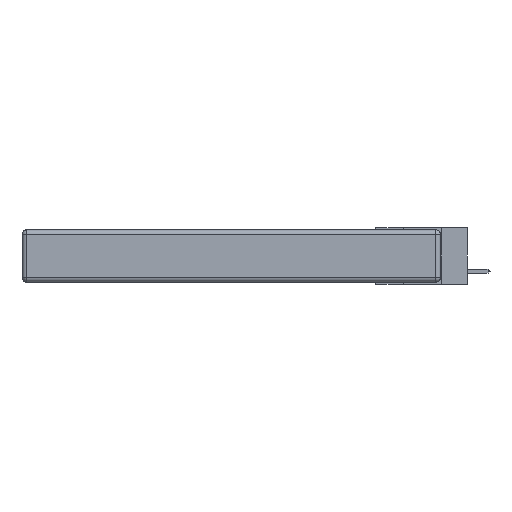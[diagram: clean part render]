
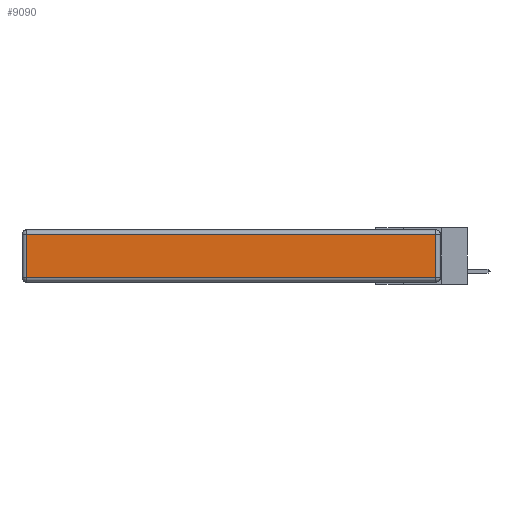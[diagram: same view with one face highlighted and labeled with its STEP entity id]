
A CAD part, left-side view. The second image highlights one B-rep face of the part: STEP entity #9090.
In plain terms, the highlighted planar face has unit normal (-1, 0, 0).
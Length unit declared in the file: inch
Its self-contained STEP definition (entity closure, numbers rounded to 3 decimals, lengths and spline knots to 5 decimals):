
#106 = CARTESIAN_POINT ( 'NONE',  ( 0., 0.03, -0.313 ) ) ;
#1104 = PLANE ( 'NONE',  #8546 ) ;
#1683 = CARTESIAN_POINT ( 'NONE',  ( 0., 2.75, -0.03 ) ) ;
#2024 = VECTOR ( 'NONE', #6876, 39.37008 ) ;
#2423 = FACE_OUTER_BOUND ( 'NONE', #12102, .T. ) ;
#2875 = CARTESIAN_POINT ( 'NONE',  ( 0., 0., -0.343 ) ) ;
#2910 = ORIENTED_EDGE ( 'NONE', *, *, #21826, .T. ) ;
#3122 = VECTOR ( 'NONE', #6326, 39.37008 ) ;
#3180 = LINE ( 'NONE', #3211, #18531 ) ;
#3211 = CARTESIAN_POINT ( 'NONE',  ( 0., 2.72, -0.343 ) ) ;
#3883 = CARTESIAN_POINT ( 'NONE',  ( 0., 2.72, -0.313 ) ) ;
#5077 = EDGE_CURVE ( 'NONE', #22896, #17038, #14555, .T. ) ;
#5767 = ORIENTED_EDGE ( 'NONE', *, *, #5077, .T. ) ;
#6326 = DIRECTION ( 'NONE',  ( 0., 0., 1. ) ) ;
#6363 = DIRECTION ( 'NONE',  ( 0., 0., 1. ) ) ;
#6567 = EDGE_CURVE ( 'NONE', #17338, #20947, #8074, .T. ) ;
#6876 = DIRECTION ( 'NONE',  ( 0., 1., 0. ) ) ;
#8074 = LINE ( 'NONE', #18659, #10877 ) ;
#8546 = AXIS2_PLACEMENT_3D ( 'NONE', #2875, #11817, #6363 ) ;
#9090 = ADVANCED_FACE ( 'NONE', ( #2423 ), #1104, .T. ) ;
#9439 = ORIENTED_EDGE ( 'NONE', *, *, #6567, .T. ) ;
#10877 = VECTOR ( 'NONE', #22487, 39.37008 ) ;
#11122 = EDGE_CURVE ( 'NONE', #20947, #22896, #17356, .T. ) ;
#11566 = CARTESIAN_POINT ( 'NONE',  ( 0., 2.72, -0.03 ) ) ;
#11817 = DIRECTION ( 'NONE',  ( -1., 0., 0. ) ) ;
#12102 = EDGE_LOOP ( 'NONE', ( #9439, #12177, #5767, #2910 ) ) ;
#12177 = ORIENTED_EDGE ( 'NONE', *, *, #11122, .T. ) ;
#12902 = CARTESIAN_POINT ( 'NONE',  ( 0., 0.03, -0.03 ) ) ;
#13655 = CARTESIAN_POINT ( 'NONE',  ( 0., 0.03, -0.343 ) ) ;
#13787 = DIRECTION ( 'NONE',  ( 0., 0., -1. ) ) ;
#14555 = LINE ( 'NONE', #1683, #2024 ) ;
#17038 = VERTEX_POINT ( 'NONE', #11566 ) ;
#17338 = VERTEX_POINT ( 'NONE', #3883 ) ;
#17356 = LINE ( 'NONE', #13655, #3122 ) ;
#18531 = VECTOR ( 'NONE', #13787, 39.37008 ) ;
#18659 = CARTESIAN_POINT ( 'NONE',  ( 0., 0., -0.313 ) ) ;
#20947 = VERTEX_POINT ( 'NONE', #106 ) ;
#21826 = EDGE_CURVE ( 'NONE', #17038, #17338, #3180, .T. ) ;
#22487 = DIRECTION ( 'NONE',  ( 0., -1., 0. ) ) ;
#22896 = VERTEX_POINT ( 'NONE', #12902 ) ;
